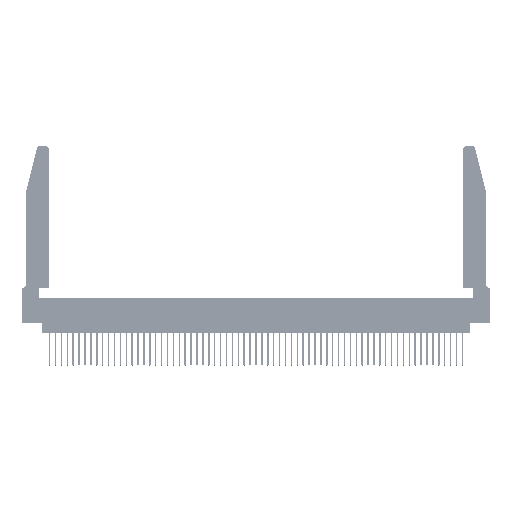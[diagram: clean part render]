
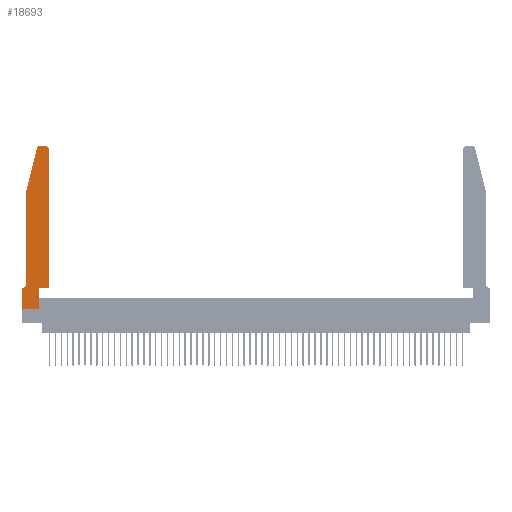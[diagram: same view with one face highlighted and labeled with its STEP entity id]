
A CAD part, top view. The second image highlights one B-rep face of the part: STEP entity #18693.
In plain terms, the highlighted planar face has unit normal (0, 0, 1).
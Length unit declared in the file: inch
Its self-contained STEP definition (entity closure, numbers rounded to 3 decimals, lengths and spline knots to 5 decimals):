
#62 = VERTEX_POINT ( 'NONE', #33906 ) ;
#185 = LINE ( 'NONE', #5121, #45592 ) ;
#1443 = VERTEX_POINT ( 'NONE', #42711 ) ;
#1815 = CARTESIAN_POINT ( 'NONE',  ( 0.25487, 2.72718, 0.37 ) ) ;
#2010 = DIRECTION ( 'NONE',  ( 1., 0., 0. ) ) ;
#2117 = CARTESIAN_POINT ( 'NONE',  ( 0.4505, 0.35, 0.37 ) ) ;
#2427 = VECTOR ( 'NONE', #6921, 39.37008 ) ;
#2691 = LINE ( 'NONE', #41647, #11686 ) ;
#3879 = EDGE_CURVE ( 'NONE', #26633, #35988, #185, .T. ) ;
#4459 = VECTOR ( 'NONE', #41360, 39.37008 ) ;
#5121 = CARTESIAN_POINT ( 'NONE',  ( 0.0755, 2., 0.37 ) ) ;
#5266 = VECTOR ( 'NONE', #16974, 39.37008 ) ;
#5412 = CARTESIAN_POINT ( 'NONE',  ( 0.0755, 0.35, 0.37 ) ) ;
#6297 = CARTESIAN_POINT ( 'NONE',  ( 0., 0.35, 0.37 ) ) ;
#6921 = DIRECTION ( 'NONE',  ( 0., -1., 0. ) ) ;
#7494 = ORIENTED_EDGE ( 'NONE', *, *, #21180, .T. ) ;
#7603 = VECTOR ( 'NONE', #36656, 39.37008 ) ;
#8072 = ORIENTED_EDGE ( 'NONE', *, *, #29535, .T. ) ;
#9767 = EDGE_CURVE ( 'NONE', #16568, #49756, #24491, .T. ) ;
#10739 = DIRECTION ( 'NONE',  ( 1., 0., 0. ) ) ;
#10922 = DIRECTION ( 'NONE',  ( -1., 0., 0. ) ) ;
#11035 = EDGE_CURVE ( 'NONE', #62, #54296, #39534, .T. ) ;
#11570 = VECTOR ( 'NONE', #17887, 39.37008 ) ;
#11686 = VECTOR ( 'NONE', #10922, 39.37008 ) ;
#14003 = CARTESIAN_POINT ( 'NONE',  ( 0.4205, 2.75, 0.37 ) ) ;
#14363 = EDGE_CURVE ( 'NONE', #31376, #43998, #22989, .T. ) ;
#14456 = CIRCLE ( 'NONE', #49438, 0.03 ) ;
#15024 = CARTESIAN_POINT ( 'NONE',  ( 0.0055, 0.42, 0.37 ) ) ;
#15052 = ORIENTED_EDGE ( 'NONE', *, *, #20164, .T. ) ;
#16568 = VERTEX_POINT ( 'NONE', #33673 ) ;
#16974 = DIRECTION ( 'NONE',  ( 1., 0., 0. ) ) ;
#17887 = DIRECTION ( 'NONE',  ( 0., -1., 0. ) ) ;
#18456 = EDGE_CURVE ( 'NONE', #35988, #31376, #24635, .T. ) ;
#18521 = ORIENTED_EDGE ( 'NONE', *, *, #44902, .T. ) ;
#18693 = ADVANCED_FACE ( 'NONE', ( #41880 ), #32474, .T. ) ;
#18810 = EDGE_LOOP ( 'NONE', ( #8072, #56631, #37631, #36979, #41091, #45204, #32944, #15052, #7494, #18521, #34370, #51344 ) ) ;
#19122 = VERTEX_POINT ( 'NONE', #49561 ) ;
#19320 = DIRECTION ( 'NONE',  ( 0., 0., 1. ) ) ;
#19432 = DIRECTION ( 'NONE',  ( -1., 0., 0. ) ) ;
#20164 = EDGE_CURVE ( 'NONE', #49756, #54044, #53220, .T. ) ;
#21180 = EDGE_CURVE ( 'NONE', #54044, #1443, #26609, .T. ) ;
#21820 = AXIS2_PLACEMENT_3D ( 'NONE', #15024, #45699, #19432 ) ;
#22498 = EDGE_CURVE ( 'NONE', #43998, #16568, #52370, .T. ) ;
#22989 = CIRCLE ( 'NONE', #21820, 0.07 ) ;
#24491 = LINE ( 'NONE', #37651, #2427 ) ;
#24635 = LINE ( 'NONE', #39751, #11570 ) ;
#26054 = CARTESIAN_POINT ( 'NONE',  ( 0.2865, 0., 0.37 ) ) ;
#26483 = VERTEX_POINT ( 'NONE', #14003 ) ;
#26609 = LINE ( 'NONE', #53582, #48475 ) ;
#26633 = VERTEX_POINT ( 'NONE', #1815 ) ;
#27057 = DIRECTION ( 'NONE',  ( -0.239, -0.971, 0. ) ) ;
#27487 = DIRECTION ( 'NONE',  ( 0., 1., 0. ) ) ;
#28429 = DIRECTION ( 'NONE',  ( 0., 0., 1. ) ) ;
#29493 = EDGE_CURVE ( 'NONE', #54296, #26483, #14456, .T. ) ;
#29535 = EDGE_CURVE ( 'NONE', #26483, #19122, #2691, .T. ) ;
#31376 = VERTEX_POINT ( 'NONE', #36102 ) ;
#31979 = EDGE_CURVE ( 'NONE', #19122, #26633, #42443, .T. ) ;
#32268 = CARTESIAN_POINT ( 'NONE',  ( 0.4505, 0.35, 0.37 ) ) ;
#32371 = LINE ( 'NONE', #32268, #7603 ) ;
#32474 = PLANE ( 'NONE',  #50159 ) ;
#32944 = ORIENTED_EDGE ( 'NONE', *, *, #9767, .T. ) ;
#33673 = CARTESIAN_POINT ( 'NONE',  ( 0., 0.35, 0.37 ) ) ;
#33906 = CARTESIAN_POINT ( 'NONE',  ( 0.4505, 0.35, 0.37 ) ) ;
#34370 = ORIENTED_EDGE ( 'NONE', *, *, #11035, .T. ) ;
#35988 = VERTEX_POINT ( 'NONE', #51589 ) ;
#36102 = CARTESIAN_POINT ( 'NONE',  ( 0.0755, 0.42, 0.37 ) ) ;
#36570 = CARTESIAN_POINT ( 'NONE',  ( 0.4505, 2.72, 0.37 ) ) ;
#36656 = DIRECTION ( 'NONE',  ( 1., 0., 0. ) ) ;
#36979 = ORIENTED_EDGE ( 'NONE', *, *, #18456, .T. ) ;
#37037 = DIRECTION ( 'NONE',  ( 0., 0., 1. ) ) ;
#37166 = CARTESIAN_POINT ( 'NONE',  ( 0., 0., 0.37 ) ) ;
#37631 = ORIENTED_EDGE ( 'NONE', *, *, #3879, .T. ) ;
#37651 = CARTESIAN_POINT ( 'NONE',  ( 0., 0., 0.37 ) ) ;
#39534 = LINE ( 'NONE', #2117, #4459 ) ;
#39751 = CARTESIAN_POINT ( 'NONE',  ( 0.0755, 2., 0.37 ) ) ;
#40576 = DIRECTION ( 'NONE',  ( -1., 0., 0. ) ) ;
#41091 = ORIENTED_EDGE ( 'NONE', *, *, #14363, .T. ) ;
#41360 = DIRECTION ( 'NONE',  ( 0., 1., 0. ) ) ;
#41647 = CARTESIAN_POINT ( 'NONE',  ( 0.2605, 2.75, 0.37 ) ) ;
#41880 = FACE_OUTER_BOUND ( 'NONE', #18810, .T. ) ;
#42443 = CIRCLE ( 'NONE', #53476, 0.03 ) ;
#42711 = CARTESIAN_POINT ( 'NONE',  ( 0.2865, 0.35, 0.37 ) ) ;
#43998 = VERTEX_POINT ( 'NONE', #46387 ) ;
#44902 = EDGE_CURVE ( 'NONE', #1443, #62, #32371, .T. ) ;
#45204 = ORIENTED_EDGE ( 'NONE', *, *, #22498, .T. ) ;
#45592 = VECTOR ( 'NONE', #27057, 39.37008 ) ;
#45596 = CARTESIAN_POINT ( 'NONE',  ( 0.284, 2.72, 0.37 ) ) ;
#45699 = DIRECTION ( 'NONE',  ( 0., 0., -1. ) ) ;
#46387 = CARTESIAN_POINT ( 'NONE',  ( 0.0055, 0.35, 0.37 ) ) ;
#48475 = VECTOR ( 'NONE', #27487, 39.37008 ) ;
#49438 = AXIS2_PLACEMENT_3D ( 'NONE', #54511, #28429, #2010 ) ;
#49561 = CARTESIAN_POINT ( 'NONE',  ( 0.284, 2.75, 0.37 ) ) ;
#49756 = VERTEX_POINT ( 'NONE', #37166 ) ;
#49906 = DIRECTION ( 'NONE',  ( 1., 0., 0. ) ) ;
#50159 = AXIS2_PLACEMENT_3D ( 'NONE', #6297, #37037, #10739 ) ;
#51344 = ORIENTED_EDGE ( 'NONE', *, *, #29493, .T. ) ;
#51589 = CARTESIAN_POINT ( 'NONE',  ( 0.0755, 2., 0.37 ) ) ;
#51892 = CARTESIAN_POINT ( 'NONE',  ( 0., 0., 0.37 ) ) ;
#52370 = LINE ( 'NONE', #5412, #53715 ) ;
#53220 = LINE ( 'NONE', #51892, #5266 ) ;
#53476 = AXIS2_PLACEMENT_3D ( 'NONE', #45596, #19320, #49906 ) ;
#53582 = CARTESIAN_POINT ( 'NONE',  ( 0.2865, 0.35, 0.37 ) ) ;
#53715 = VECTOR ( 'NONE', #40576, 39.37008 ) ;
#54044 = VERTEX_POINT ( 'NONE', #26054 ) ;
#54296 = VERTEX_POINT ( 'NONE', #36570 ) ;
#54511 = CARTESIAN_POINT ( 'NONE',  ( 0.4205, 2.72, 0.37 ) ) ;
#56631 = ORIENTED_EDGE ( 'NONE', *, *, #31979, .T. ) ;
